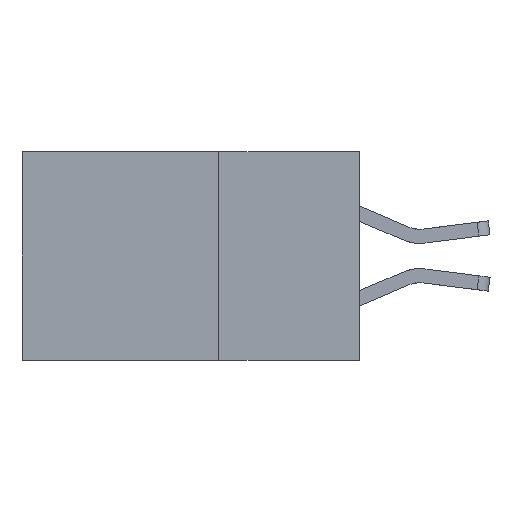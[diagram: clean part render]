
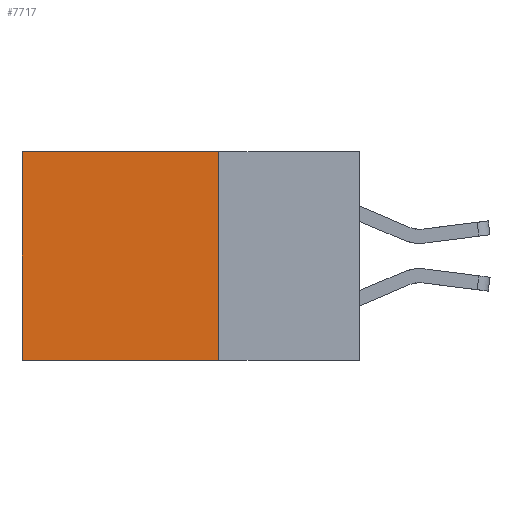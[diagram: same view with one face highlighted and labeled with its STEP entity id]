
A CAD part, left-side view. The second image highlights one B-rep face of the part: STEP entity #7717.
In plain terms, the highlighted planar face has unit normal (-1, 0, 0).
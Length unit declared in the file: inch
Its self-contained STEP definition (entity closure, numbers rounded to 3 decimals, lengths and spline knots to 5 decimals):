
#33 = CARTESIAN_POINT ( 'NONE',  ( 0.2875, 0.25, -0.37 ) ) ;
#107 = CARTESIAN_POINT ( 'NONE',  ( 0.2875, 0.25, 0. ) ) ;
#557 = ORIENTED_EDGE ( 'NONE', *, *, #10895, .F. ) ;
#692 = DIRECTION ( 'NONE',  ( 0., 0., -1. ) ) ;
#828 = DIRECTION ( 'NONE',  ( 0., 1., 0. ) ) ;
#948 = PLANE ( 'NONE',  #10329 ) ;
#1122 = CARTESIAN_POINT ( 'NONE',  ( 0.2875, 0.6, -0.37 ) ) ;
#1373 = EDGE_CURVE ( 'NONE', #10104, #10643, #10758, .T. ) ;
#1375 = VECTOR ( 'NONE', #828, 39.37008 ) ;
#1911 = FACE_OUTER_BOUND ( 'NONE', #8714, .T. ) ;
#1922 = DIRECTION ( 'NONE',  ( 1., 0., 0. ) ) ;
#1976 = ORIENTED_EDGE ( 'NONE', *, *, #1373, .F. ) ;
#2244 = CARTESIAN_POINT ( 'NONE',  ( 0.2875, 0.25, -0.37 ) ) ;
#2799 = CARTESIAN_POINT ( 'NONE',  ( 0.2875, 0.25, 0. ) ) ;
#3048 = VERTEX_POINT ( 'NONE', #1122 ) ;
#3392 = VECTOR ( 'NONE', #692, 39.37008 ) ;
#3688 = ORIENTED_EDGE ( 'NONE', *, *, #4189, .T. ) ;
#3846 = CARTESIAN_POINT ( 'NONE',  ( 0.2875, 0.25, 0. ) ) ;
#4189 = EDGE_CURVE ( 'NONE', #9790, #3048, #7628, .T. ) ;
#4801 = DIRECTION ( 'NONE',  ( 0., 0., -1. ) ) ;
#5265 = VECTOR ( 'NONE', #4801, 39.37008 ) ;
#5363 = ORIENTED_EDGE ( 'NONE', *, *, #11327, .T. ) ;
#6254 = CARTESIAN_POINT ( 'NONE',  ( 0.2875, 0.25, 0. ) ) ;
#7628 = LINE ( 'NONE', #8357, #5265 ) ;
#7717 = ADVANCED_FACE ( 'NONE', ( #1911 ), #948, .F. ) ;
#8186 = DIRECTION ( 'NONE',  ( 0., 0., -1. ) ) ;
#8357 = CARTESIAN_POINT ( 'NONE',  ( 0.2875, 0.6, 0. ) ) ;
#8534 = DIRECTION ( 'NONE',  ( 0., 1., 0. ) ) ;
#8557 = LINE ( 'NONE', #6254, #1375 ) ;
#8714 = EDGE_LOOP ( 'NONE', ( #3688, #557, #1976, #5363 ) ) ;
#9679 = CARTESIAN_POINT ( 'NONE',  ( 0.2875, 0.6, 0. ) ) ;
#9790 = VERTEX_POINT ( 'NONE', #9679 ) ;
#10104 = VERTEX_POINT ( 'NONE', #3846 ) ;
#10329 = AXIS2_PLACEMENT_3D ( 'NONE', #2799, #1922, #8186 ) ;
#10643 = VERTEX_POINT ( 'NONE', #33 ) ;
#10663 = VECTOR ( 'NONE', #8534, 39.37008 ) ;
#10758 = LINE ( 'NONE', #107, #3392 ) ;
#10895 = EDGE_CURVE ( 'NONE', #10643, #3048, #10948, .T. ) ;
#10948 = LINE ( 'NONE', #2244, #10663 ) ;
#11327 = EDGE_CURVE ( 'NONE', #10104, #9790, #8557, .T. ) ;
